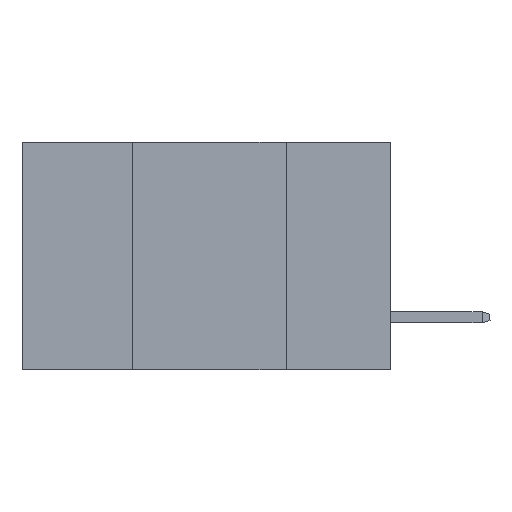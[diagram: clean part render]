
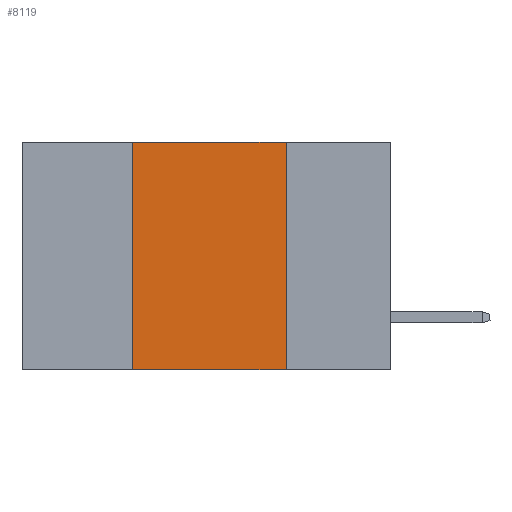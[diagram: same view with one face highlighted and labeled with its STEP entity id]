
A CAD part, left-side view. The second image highlights one B-rep face of the part: STEP entity #8119.
In plain terms, the highlighted planar face has unit normal (-1, 0, 0).
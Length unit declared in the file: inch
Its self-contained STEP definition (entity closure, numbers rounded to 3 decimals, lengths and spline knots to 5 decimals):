
#277 = CARTESIAN_POINT ( 'NONE',  ( 0., 0.42, 0. ) ) ;
#513 = VECTOR ( 'NONE', #1923, 39.37008 ) ;
#782 = CARTESIAN_POINT ( 'NONE',  ( 0., 0.6, 0. ) ) ;
#1059 = ORIENTED_EDGE ( 'NONE', *, *, #5649, .T. ) ;
#1134 = LINE ( 'NONE', #6118, #8414 ) ;
#1161 = DIRECTION ( 'NONE',  ( 0., 0., -1. ) ) ;
#1283 = VECTOR ( 'NONE', #9024, 39.37008 ) ;
#1430 = VERTEX_POINT ( 'NONE', #7265 ) ;
#1480 = EDGE_CURVE ( 'NONE', #5767, #3268, #3956, .T. ) ;
#1923 = DIRECTION ( 'NONE',  ( 0., 0., 1. ) ) ;
#2805 = VECTOR ( 'NONE', #6642, 39.37008 ) ;
#3268 = VERTEX_POINT ( 'NONE', #5459 ) ;
#3490 = LINE ( 'NONE', #782, #1283 ) ;
#3713 = VERTEX_POINT ( 'NONE', #8998 ) ;
#3956 = LINE ( 'NONE', #5003, #2805 ) ;
#4583 = PLANE ( 'NONE',  #8798 ) ;
#4639 = EDGE_CURVE ( 'NONE', #3713, #5767, #3490, .T. ) ;
#5003 = CARTESIAN_POINT ( 'NONE',  ( 0., 0.17, 0. ) ) ;
#5459 = CARTESIAN_POINT ( 'NONE',  ( 0., 0.17, -0.37 ) ) ;
#5649 = EDGE_CURVE ( 'NONE', #1430, #3268, #1134, .T. ) ;
#5767 = VERTEX_POINT ( 'NONE', #7293 ) ;
#5932 = ORIENTED_EDGE ( 'NONE', *, *, #4639, .F. ) ;
#6118 = CARTESIAN_POINT ( 'NONE',  ( 0., 0.6, -0.37 ) ) ;
#6285 = ORIENTED_EDGE ( 'NONE', *, *, #1480, .F. ) ;
#6642 = DIRECTION ( 'NONE',  ( 0., 0., -1. ) ) ;
#7172 = EDGE_LOOP ( 'NONE', ( #6285, #5932, #10715, #1059 ) ) ;
#7265 = CARTESIAN_POINT ( 'NONE',  ( 0., 0.42, -0.37 ) ) ;
#7293 = CARTESIAN_POINT ( 'NONE',  ( 0., 0.17, 0. ) ) ;
#8119 = ADVANCED_FACE ( 'NONE', ( #9147 ), #4583, .F. ) ;
#8414 = VECTOR ( 'NONE', #9471, 39.37008 ) ;
#8798 = AXIS2_PLACEMENT_3D ( 'NONE', #9630, #10338, #1161 ) ;
#8998 = CARTESIAN_POINT ( 'NONE',  ( 0., 0.42, 0. ) ) ;
#9024 = DIRECTION ( 'NONE',  ( 0., -1., 0. ) ) ;
#9147 = FACE_OUTER_BOUND ( 'NONE', #7172, .T. ) ;
#9440 = EDGE_CURVE ( 'NONE', #1430, #3713, #10574, .T. ) ;
#9471 = DIRECTION ( 'NONE',  ( 0., -1., 0. ) ) ;
#9630 = CARTESIAN_POINT ( 'NONE',  ( 0., 0.6, 0. ) ) ;
#10338 = DIRECTION ( 'NONE',  ( 1., 0., 0. ) ) ;
#10574 = LINE ( 'NONE', #277, #513 ) ;
#10715 = ORIENTED_EDGE ( 'NONE', *, *, #9440, .F. ) ;
